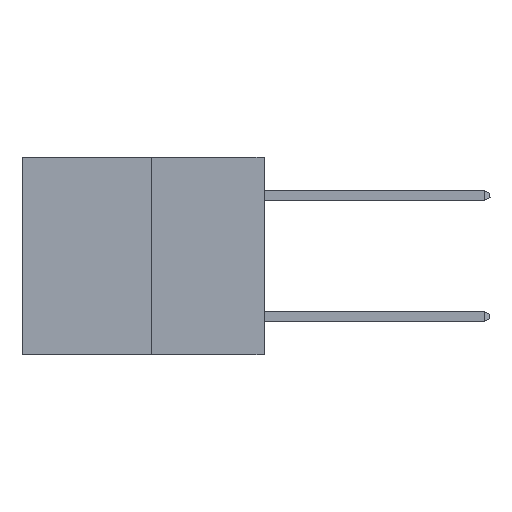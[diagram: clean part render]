
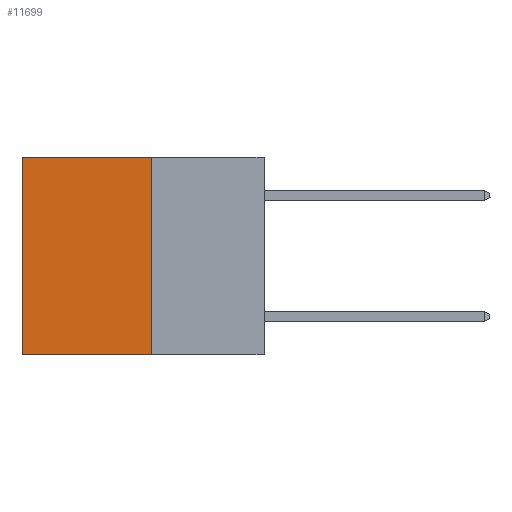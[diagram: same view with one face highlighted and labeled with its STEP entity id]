
A CAD part, left-side view. The second image highlights one B-rep face of the part: STEP entity #11699.
In plain terms, the highlighted planar face has unit normal (-1, 0, 0).
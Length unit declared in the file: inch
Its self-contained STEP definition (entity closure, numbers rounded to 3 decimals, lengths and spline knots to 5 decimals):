
#693 = LINE ( 'NONE', #4052, #15760 ) ;
#2017 = DIRECTION ( 'NONE',  ( 0., 0., -1. ) ) ;
#4052 = CARTESIAN_POINT ( 'NONE',  ( 0.3165, 0.28, 0. ) ) ;
#4516 = ORIENTED_EDGE ( 'NONE', *, *, #24829, .T. ) ;
#4957 = CARTESIAN_POINT ( 'NONE',  ( 0.3165, 0.6, -0.49 ) ) ;
#5998 = DIRECTION ( 'NONE',  ( 0., 1., 0. ) ) ;
#6382 = EDGE_LOOP ( 'NONE', ( #24691, #17083, #19997, #4516 ) ) ;
#6819 = CARTESIAN_POINT ( 'NONE',  ( 0.3165, 0.28, -0.49 ) ) ;
#8609 = CARTESIAN_POINT ( 'NONE',  ( 0.3165, 0.6, 0. ) ) ;
#10250 = EDGE_CURVE ( 'NONE', #17893, #10612, #11917, .T. ) ;
#10612 = VERTEX_POINT ( 'NONE', #11549 ) ;
#11549 = CARTESIAN_POINT ( 'NONE',  ( 0.3165, 0.6, -0.49 ) ) ;
#11576 = AXIS2_PLACEMENT_3D ( 'NONE', #23028, #13074, #19050 ) ;
#11699 = ADVANCED_FACE ( 'NONE', ( #15166 ), #22780, .F. ) ;
#11917 = LINE ( 'NONE', #4957, #24355 ) ;
#11991 = LINE ( 'NONE', #13867, #19034 ) ;
#12158 = VECTOR ( 'NONE', #2017, 39.37008 ) ;
#12316 = CARTESIAN_POINT ( 'NONE',  ( 0.3165, 0.28, 0. ) ) ;
#13074 = DIRECTION ( 'NONE',  ( 1., 0., 0. ) ) ;
#13867 = CARTESIAN_POINT ( 'NONE',  ( 0.3165, 0.28, -0.49 ) ) ;
#14600 = LINE ( 'NONE', #21074, #12158 ) ;
#15166 = FACE_OUTER_BOUND ( 'NONE', #6382, .T. ) ;
#15760 = VECTOR ( 'NONE', #5998, 39.37008 ) ;
#16732 = EDGE_CURVE ( 'NONE', #19396, #10612, #11991, .T. ) ;
#17083 = ORIENTED_EDGE ( 'NONE', *, *, #16732, .F. ) ;
#17893 = VERTEX_POINT ( 'NONE', #8609 ) ;
#18807 = VERTEX_POINT ( 'NONE', #12316 ) ;
#19034 = VECTOR ( 'NONE', #21760, 39.37008 ) ;
#19050 = DIRECTION ( 'NONE',  ( 0., 0., -1. ) ) ;
#19073 = EDGE_CURVE ( 'NONE', #18807, #19396, #14600, .T. ) ;
#19396 = VERTEX_POINT ( 'NONE', #6819 ) ;
#19997 = ORIENTED_EDGE ( 'NONE', *, *, #19073, .F. ) ;
#21074 = CARTESIAN_POINT ( 'NONE',  ( 0.3165, 0.28, -0.49 ) ) ;
#21760 = DIRECTION ( 'NONE',  ( 0., 1., 0. ) ) ;
#22403 = DIRECTION ( 'NONE',  ( 0., 0., -1. ) ) ;
#22780 = PLANE ( 'NONE',  #11576 ) ;
#23028 = CARTESIAN_POINT ( 'NONE',  ( 0.3165, 0.28, -0.49 ) ) ;
#24355 = VECTOR ( 'NONE', #22403, 39.37008 ) ;
#24691 = ORIENTED_EDGE ( 'NONE', *, *, #10250, .T. ) ;
#24829 = EDGE_CURVE ( 'NONE', #18807, #17893, #693, .T. ) ;
